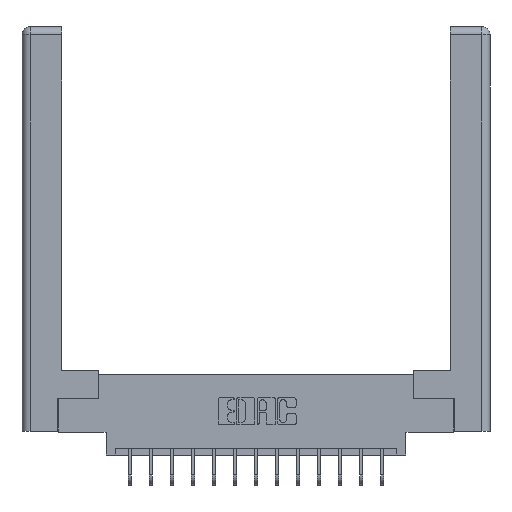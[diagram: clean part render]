
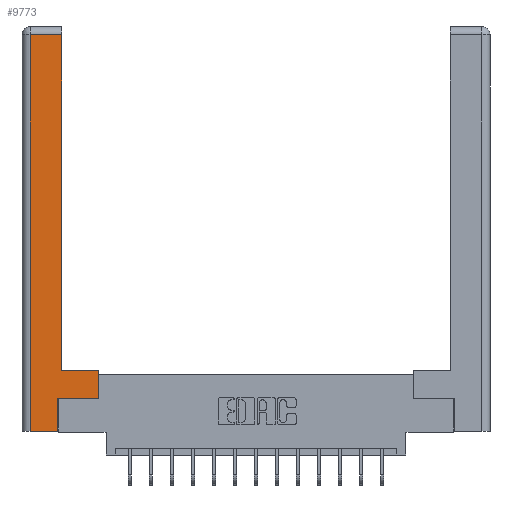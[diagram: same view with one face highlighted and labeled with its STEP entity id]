
A CAD part, top view. The second image highlights one B-rep face of the part: STEP entity #9773.
In plain terms, the highlighted planar face has unit normal (0, 0, 1).
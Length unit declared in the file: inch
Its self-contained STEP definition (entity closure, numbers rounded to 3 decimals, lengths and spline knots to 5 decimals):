
#227 = VERTEX_POINT ( 'NONE', #15189 ) ;
#547 = EDGE_CURVE ( 'NONE', #1597, #5100, #2985, .T. ) ;
#989 = CARTESIAN_POINT ( 'NONE',  ( 0.295, 0.45, 0. ) ) ;
#1294 = AXIS2_PLACEMENT_3D ( 'NONE', #12211, #3746, #13659 ) ;
#1465 = EDGE_CURVE ( 'NONE', #7486, #2811, #9369, .T. ) ;
#1597 = VERTEX_POINT ( 'NONE', #1825 ) ;
#1793 = EDGE_CURVE ( 'NONE', #5100, #227, #16236, .T. ) ;
#1825 = CARTESIAN_POINT ( 'NONE',  ( 0.565, 0.45, 0. ) ) ;
#2455 = EDGE_LOOP ( 'NONE', ( #13496, #16248, #16878, #16556, #15597, #14962, #17223, #3751 ) ) ;
#2811 = VERTEX_POINT ( 'NONE', #4889 ) ;
#2952 = EDGE_CURVE ( 'NONE', #15709, #15896, #7570, .T. ) ;
#2985 = LINE ( 'NONE', #4736, #17857 ) ;
#3046 = VECTOR ( 'NONE', #4193, 39.37008 ) ;
#3746 = DIRECTION ( 'NONE',  ( 0., 0., -1. ) ) ;
#3751 = ORIENTED_EDGE ( 'NONE', *, *, #547, .T. ) ;
#3826 = CARTESIAN_POINT ( 'NONE',  ( 0.0615, 2.94, 0. ) ) ;
#3863 = CARTESIAN_POINT ( 'NONE',  ( 0.295, 3., 0. ) ) ;
#4193 = DIRECTION ( 'NONE',  ( 1., 0., 0. ) ) ;
#4245 = DIRECTION ( 'NONE',  ( 0., -1., 0. ) ) ;
#4736 = CARTESIAN_POINT ( 'NONE',  ( 0.295, 0.45, 0. ) ) ;
#4889 = CARTESIAN_POINT ( 'NONE',  ( 0.0615, 0., 0. ) ) ;
#5100 = VERTEX_POINT ( 'NONE', #989 ) ;
#5184 = PLANE ( 'NONE',  #1294 ) ;
#5932 = CARTESIAN_POINT ( 'NONE',  ( 0.565, 0.245, 0. ) ) ;
#6188 = DIRECTION ( 'NONE',  ( -1., 0., 0. ) ) ;
#7125 = VECTOR ( 'NONE', #9981, 39.37008 ) ;
#7201 = FACE_OUTER_BOUND ( 'NONE', #2455, .T. ) ;
#7231 = LINE ( 'NONE', #17101, #8345 ) ;
#7486 = VERTEX_POINT ( 'NONE', #3826 ) ;
#7570 = LINE ( 'NONE', #5932, #7125 ) ;
#7695 = VECTOR ( 'NONE', #7911, 39.37008 ) ;
#7911 = DIRECTION ( 'NONE',  ( -1., 0., 0. ) ) ;
#8086 = CARTESIAN_POINT ( 'NONE',  ( 0.0615, 2.94, 0. ) ) ;
#8345 = VECTOR ( 'NONE', #8589, 39.37008 ) ;
#8589 = DIRECTION ( 'NONE',  ( 0., 1., 0. ) ) ;
#8726 = EDGE_CURVE ( 'NONE', #2811, #10793, #10352, .T. ) ;
#9193 = VECTOR ( 'NONE', #13831, 39.37008 ) ;
#9369 = LINE ( 'NONE', #11525, #12461 ) ;
#9773 = ADVANCED_FACE ( 'NONE', ( #7201 ), #5184, .F. ) ;
#9981 = DIRECTION ( 'NONE',  ( 1., 0., 0. ) ) ;
#10264 = CARTESIAN_POINT ( 'NONE',  ( 0.565, 0.245, 0. ) ) ;
#10352 = LINE ( 'NONE', #12356, #3046 ) ;
#10793 = VERTEX_POINT ( 'NONE', #14619 ) ;
#10800 = DIRECTION ( 'NONE',  ( 0., 1., 0. ) ) ;
#11525 = CARTESIAN_POINT ( 'NONE',  ( 0.0615, 0., 0. ) ) ;
#12211 = CARTESIAN_POINT ( 'NONE',  ( 0., 0., 0. ) ) ;
#12356 = CARTESIAN_POINT ( 'NONE',  ( 0.265, 0., 0. ) ) ;
#12389 = CARTESIAN_POINT ( 'NONE',  ( 0.265, 0.245, 0. ) ) ;
#12461 = VECTOR ( 'NONE', #4245, 39.37008 ) ;
#13496 = ORIENTED_EDGE ( 'NONE', *, *, #1793, .T. ) ;
#13659 = DIRECTION ( 'NONE',  ( -1., 0., 0. ) ) ;
#13831 = DIRECTION ( 'NONE',  ( 0., 1., 0. ) ) ;
#14438 = EDGE_CURVE ( 'NONE', #227, #7486, #17470, .T. ) ;
#14619 = CARTESIAN_POINT ( 'NONE',  ( 0.265, 0., 0. ) ) ;
#14897 = VECTOR ( 'NONE', #10800, 39.37008 ) ;
#14962 = ORIENTED_EDGE ( 'NONE', *, *, #2952, .T. ) ;
#15189 = CARTESIAN_POINT ( 'NONE',  ( 0.295, 2.94, 0. ) ) ;
#15397 = EDGE_CURVE ( 'NONE', #15896, #1597, #7231, .T. ) ;
#15597 = ORIENTED_EDGE ( 'NONE', *, *, #17151, .T. ) ;
#15709 = VERTEX_POINT ( 'NONE', #16861 ) ;
#15896 = VERTEX_POINT ( 'NONE', #10264 ) ;
#16236 = LINE ( 'NONE', #3863, #14897 ) ;
#16248 = ORIENTED_EDGE ( 'NONE', *, *, #14438, .T. ) ;
#16556 = ORIENTED_EDGE ( 'NONE', *, *, #8726, .T. ) ;
#16861 = CARTESIAN_POINT ( 'NONE',  ( 0.265, 0.245, 0. ) ) ;
#16878 = ORIENTED_EDGE ( 'NONE', *, *, #1465, .T. ) ;
#17101 = CARTESIAN_POINT ( 'NONE',  ( 0.565, 0.45, 0. ) ) ;
#17151 = EDGE_CURVE ( 'NONE', #10793, #15709, #18094, .T. ) ;
#17223 = ORIENTED_EDGE ( 'NONE', *, *, #15397, .T. ) ;
#17470 = LINE ( 'NONE', #8086, #7695 ) ;
#17857 = VECTOR ( 'NONE', #6188, 39.37008 ) ;
#18094 = LINE ( 'NONE', #12389, #9193 ) ;
